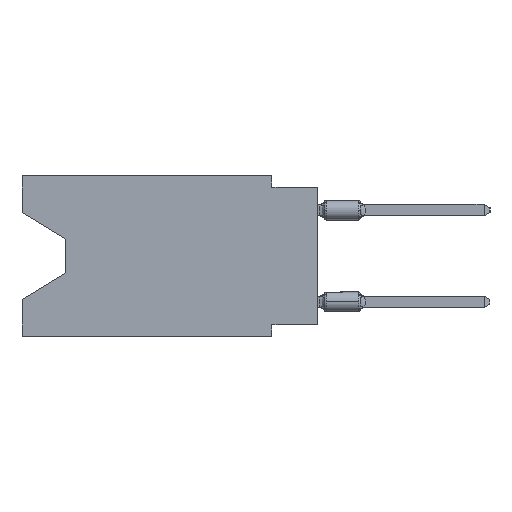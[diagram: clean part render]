
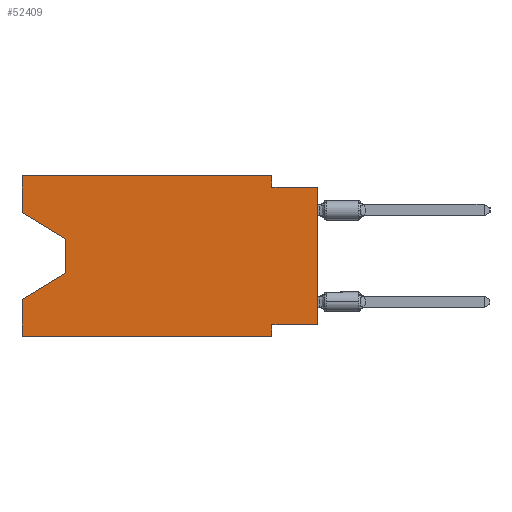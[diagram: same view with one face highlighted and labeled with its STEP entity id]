
A CAD part, left-side view. The second image highlights one B-rep face of the part: STEP entity #52409.
In plain terms, the highlighted planar face has unit normal (-1, 0, 0).
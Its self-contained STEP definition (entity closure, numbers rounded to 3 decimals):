
#1542 = ORIENTED_EDGE ( 'NONE', *, *, #26331, .F. ) ;
#2247 = VECTOR ( 'NONE', #24776, 1000. ) ;
#2468 = VECTOR ( 'NONE', #45103, 1000. ) ;
#2703 = CARTESIAN_POINT ( 'NONE',  ( 0., 13.97, -5.385 ) ) ;
#2721 = LINE ( 'NONE', #24697, #39729 ) ;
#2815 = ORIENTED_EDGE ( 'NONE', *, *, #7231, .F. ) ;
#3752 = VERTEX_POINT ( 'NONE', #8948 ) ;
#3981 = VERTEX_POINT ( 'NONE', #7466 ) ;
#4296 = ORIENTED_EDGE ( 'NONE', *, *, #24551, .T. ) ;
#4471 = EDGE_CURVE ( 'NONE', #30197, #3752, #2721, .T. ) ;
#4995 = CARTESIAN_POINT ( 'NONE',  ( 0., 16.383, 0. ) ) ;
#6344 = ORIENTED_EDGE ( 'NONE', *, *, #46117, .T. ) ;
#6387 = DIRECTION ( 'NONE',  ( 0., 0., -1. ) ) ;
#7231 = EDGE_CURVE ( 'NONE', #23337, #3981, #9394, .T. ) ;
#7466 = CARTESIAN_POINT ( 'NONE',  ( 0., 0., -0.635 ) ) ;
#8452 = LINE ( 'NONE', #26326, #37218 ) ;
#8522 = VECTOR ( 'NONE', #11840, 1000. ) ;
#8948 = CARTESIAN_POINT ( 'NONE',  ( 0., 2.54, -8.89 ) ) ;
#9144 = ORIENTED_EDGE ( 'NONE', *, *, #18285, .T. ) ;
#9394 = LINE ( 'NONE', #54453, #2468 ) ;
#10851 = CARTESIAN_POINT ( 'NONE',  ( 0., 13.97, -3.505 ) ) ;
#11359 = LINE ( 'NONE', #28960, #56454 ) ;
#11605 = ORIENTED_EDGE ( 'NONE', *, *, #48247, .F. ) ;
#11771 = DIRECTION ( 'NONE',  ( 0., 0.855, -0.519 ) ) ;
#11840 = DIRECTION ( 'NONE',  ( 0., 0., -1. ) ) ;
#11964 = VERTEX_POINT ( 'NONE', #55180 ) ;
#11999 = CARTESIAN_POINT ( 'NONE',  ( 0., 16.383, 0. ) ) ;
#12082 = DIRECTION ( 'NONE',  ( 0., -1., 0. ) ) ;
#12677 = VERTEX_POINT ( 'NONE', #14684 ) ;
#13214 = LINE ( 'NONE', #4995, #25914 ) ;
#14270 = ORIENTED_EDGE ( 'NONE', *, *, #4471, .T. ) ;
#14632 = EDGE_CURVE ( 'NONE', #35002, #47097, #13214, .T. ) ;
#14684 = CARTESIAN_POINT ( 'NONE',  ( 0., 0., -8.255 ) ) ;
#16425 = DIRECTION ( 'NONE',  ( 0., 0., -1. ) ) ;
#16957 = DIRECTION ( 'NONE',  ( 0., 0., 1. ) ) ;
#17390 = VECTOR ( 'NONE', #25997, 1000. ) ;
#17915 = DIRECTION ( 'NONE',  ( 0., 0., 1. ) ) ;
#18285 = EDGE_CURVE ( 'NONE', #35002, #51091, #8452, .T. ) ;
#22156 = VECTOR ( 'NONE', #41212, 1000. ) ;
#22996 = AXIS2_PLACEMENT_3D ( 'NONE', #11999, #24913, #16425 ) ;
#23337 = VERTEX_POINT ( 'NONE', #26030 ) ;
#24168 = CARTESIAN_POINT ( 'NONE',  ( 0., 16.383, 0. ) ) ;
#24201 = LINE ( 'NONE', #37363, #2247 ) ;
#24399 = ORIENTED_EDGE ( 'NONE', *, *, #29511, .F. ) ;
#24551 = EDGE_CURVE ( 'NONE', #11964, #46370, #29087, .T. ) ;
#24697 = CARTESIAN_POINT ( 'NONE',  ( 0., 16.383, -8.89 ) ) ;
#24776 = DIRECTION ( 'NONE',  ( 0., 0., 1. ) ) ;
#24913 = DIRECTION ( 'NONE',  ( 1., 0., 0. ) ) ;
#25914 = VECTOR ( 'NONE', #17915, 1000. ) ;
#25997 = DIRECTION ( 'NONE',  ( 0., 1., 0. ) ) ;
#26024 = LINE ( 'NONE', #29842, #47379 ) ;
#26030 = CARTESIAN_POINT ( 'NONE',  ( 0., 2.54, -0.635 ) ) ;
#26326 = CARTESIAN_POINT ( 'NONE',  ( 0., 16.383, -2.038 ) ) ;
#26331 = EDGE_CURVE ( 'NONE', #47097, #44873, #51076, .T. ) ;
#28960 = CARTESIAN_POINT ( 'NONE',  ( 0., 13.97, -3.505 ) ) ;
#29087 = LINE ( 'NONE', #2703, #29115 ) ;
#29115 = VECTOR ( 'NONE', #11771, 1000. ) ;
#29511 = EDGE_CURVE ( 'NONE', #12677, #38457, #30381, .T. ) ;
#29598 = PLANE ( 'NONE',  #22996 ) ;
#29842 = CARTESIAN_POINT ( 'NONE',  ( 0., 0., 0. ) ) ;
#30197 = VERTEX_POINT ( 'NONE', #41992 ) ;
#30381 = LINE ( 'NONE', #34189, #17390 ) ;
#30538 = ORIENTED_EDGE ( 'NONE', *, *, #46348, .F. ) ;
#30605 = VECTOR ( 'NONE', #51921, 1000. ) ;
#33878 = CARTESIAN_POINT ( 'NONE',  ( 0., 2.54, 0. ) ) ;
#34189 = CARTESIAN_POINT ( 'NONE',  ( 0., 0., -8.255 ) ) ;
#34670 = CARTESIAN_POINT ( 'NONE',  ( 0., 2.54, -8.89 ) ) ;
#35002 = VERTEX_POINT ( 'NONE', #45633 ) ;
#37218 = VECTOR ( 'NONE', #44154, 1000. ) ;
#37363 = CARTESIAN_POINT ( 'NONE',  ( 0., 16.383, 0. ) ) ;
#38457 = VERTEX_POINT ( 'NONE', #47156 ) ;
#39729 = VECTOR ( 'NONE', #12082, 1000. ) ;
#41212 = DIRECTION ( 'NONE',  ( 0., 0., -1. ) ) ;
#41983 = EDGE_CURVE ( 'NONE', #51091, #11964, #11359, .T. ) ;
#41992 = CARTESIAN_POINT ( 'NONE',  ( 0., 16.383, -8.89 ) ) ;
#43045 = FACE_OUTER_BOUND ( 'NONE', #51369, .T. ) ;
#43715 = ORIENTED_EDGE ( 'NONE', *, *, #57775, .F. ) ;
#44154 = DIRECTION ( 'NONE',  ( 0., -0.855, -0.519 ) ) ;
#44873 = VERTEX_POINT ( 'NONE', #33878 ) ;
#45103 = DIRECTION ( 'NONE',  ( 0., -1., 0. ) ) ;
#45581 = CARTESIAN_POINT ( 'NONE',  ( 0., 2.54, 0. ) ) ;
#45633 = CARTESIAN_POINT ( 'NONE',  ( 0., 16.383, -2.038 ) ) ;
#46117 = EDGE_CURVE ( 'NONE', #12677, #3981, #26024, .T. ) ;
#46348 = EDGE_CURVE ( 'NONE', #44873, #23337, #49096, .T. ) ;
#46370 = VERTEX_POINT ( 'NONE', #56024 ) ;
#47097 = VERTEX_POINT ( 'NONE', #50364 ) ;
#47156 = CARTESIAN_POINT ( 'NONE',  ( 0., 2.54, -8.255 ) ) ;
#47379 = VECTOR ( 'NONE', #16957, 1000. ) ;
#48023 = ORIENTED_EDGE ( 'NONE', *, *, #14632, .F. ) ;
#48247 = EDGE_CURVE ( 'NONE', #38457, #3752, #51931, .T. ) ;
#49096 = LINE ( 'NONE', #45581, #22156 ) ;
#49956 = ORIENTED_EDGE ( 'NONE', *, *, #41983, .T. ) ;
#50364 = CARTESIAN_POINT ( 'NONE',  ( 0., 16.383, 0. ) ) ;
#51076 = LINE ( 'NONE', #24168, #30605 ) ;
#51091 = VERTEX_POINT ( 'NONE', #10851 ) ;
#51369 = EDGE_LOOP ( 'NONE', ( #9144, #49956, #4296, #43715, #14270, #11605, #24399, #6344, #2815, #30538, #1542, #48023 ) ) ;
#51921 = DIRECTION ( 'NONE',  ( 0., -1., 0. ) ) ;
#51931 = LINE ( 'NONE', #34670, #8522 ) ;
#52409 = ADVANCED_FACE ( 'NONE', ( #43045 ), #29598, .F. ) ;
#54453 = CARTESIAN_POINT ( 'NONE',  ( 0., 0., -0.635 ) ) ;
#55180 = CARTESIAN_POINT ( 'NONE',  ( 0., 13.97, -5.385 ) ) ;
#56024 = CARTESIAN_POINT ( 'NONE',  ( 0., 16.383, -6.852 ) ) ;
#56454 = VECTOR ( 'NONE', #6387, 1000. ) ;
#57775 = EDGE_CURVE ( 'NONE', #30197, #46370, #24201, .T. ) ;
